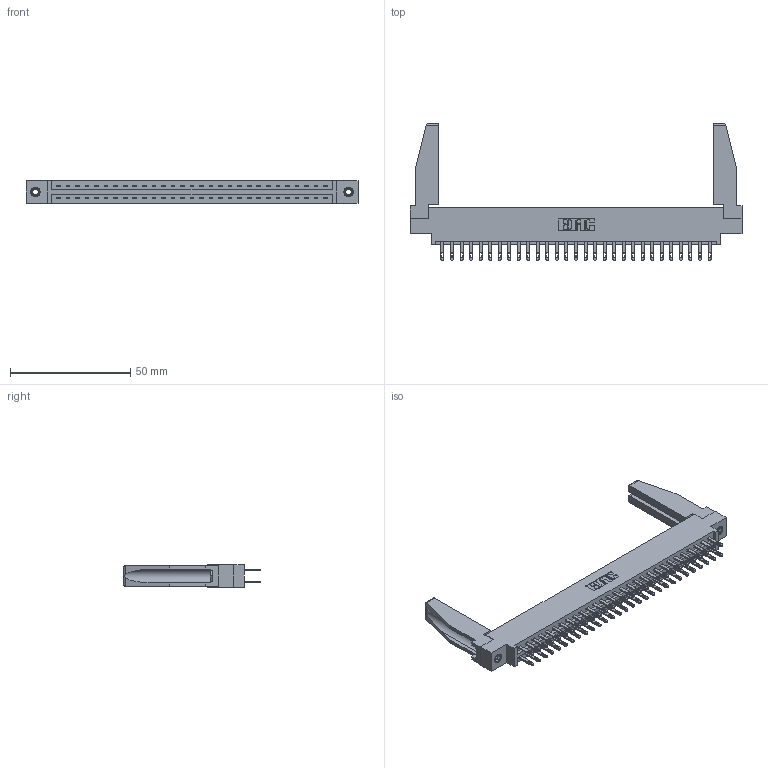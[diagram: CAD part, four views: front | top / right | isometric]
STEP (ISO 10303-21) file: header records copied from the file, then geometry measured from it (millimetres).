
FILE_DESCRIPTION (( 'STEP AP203' ), '1' );
FILE_NAME ('337-058-500-878.STEP', '2019-10-11T20:24:05', ( '' ), ( '' ), 'SwSTEP 2.0', 'SolidWorks 2016', '' );
FILE_SCHEMA (( 'CONFIG_CONTROL_DESIGN' ));
Length unit declared in the file: inch
Products named in the file (5): 345-292-001_345-293-100; 337 Part_0.170 Offset - 0.156 Dia-TI; 307-220-078; 345-250-001_345-250-001-102; 337-058-500-878
Assembly tree (63 placements, depth 2):
  337-058-500-878
    337 Part_0.170 Offset - 0.156 Dia-TI
    345-292-001_345-293-100  x58
    345-250-001_345-250-001-102  x2
    307-220-078  x2
Bounding box: 137.92 x 56.65 x 9.4 mm (x, y, z)
Volume: 18415.3 mm3; surface area: 20759.7 mm2
Topology: 63 solids, 63 shells, 3148 faces, 9527 edges, 6342 vertices
Faces by surface type: plane 2014, cylinder 1118, cone 12, torus 4
Entity records: 26668 total; most frequent: CARTESIAN_POINT 4504, ORIENTED_EDGE 4396, DIRECTION 3862, EDGE_CURVE 2198, VECTOR 2028, LINE 2028, VERTEX_POINT 1460, AXIS2_PLACEMENT_3D 917
